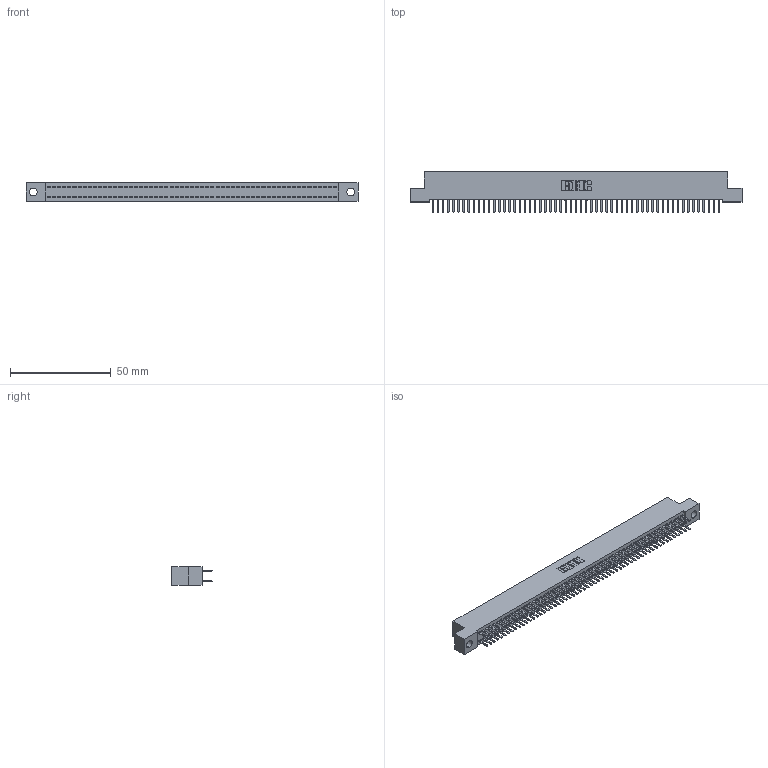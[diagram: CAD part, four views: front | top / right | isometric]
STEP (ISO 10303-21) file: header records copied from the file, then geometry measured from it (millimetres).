
FILE_DESCRIPTION (( 'STEP AP203' ), '1' );
FILE_NAME ('392-114-520-204.STEP', '2019-10-10T00:49:31', ( '' ), ( '' ), 'SwSTEP 2.0', 'SolidWorks 2016', '' );
FILE_SCHEMA (( 'CONFIG_CONTROL_DESIGN' ));
Length unit declared in the file: inch
Products named in the file (3): 392-114-520-204; 342 Part_.156 TH; 345-292-001_345-293-120
Assembly tree (115 placements, depth 2):
  392-114-520-204
    342 Part_.156 TH
    345-292-001_345-293-120  x114
Bounding box: 165.1 x 20.02 x 9.4 mm (x, y, z)
Volume: 14768.1 mm3; surface area: 24114.3 mm2
Topology: 115 solids, 115 shells, 6494 faces, 18881 edges, 12282 vertices
Faces by surface type: plane 4398, cylinder 2096
Entity records: 34715 total; most frequent: CARTESIAN_POINT 5746, ORIENTED_EDGE 5670, DIRECTION 4871, EDGE_CURVE 2835, VECTOR 2703, LINE 2703, VERTEX_POINT 1886, AXIS2_PLACEMENT_3D 1084
